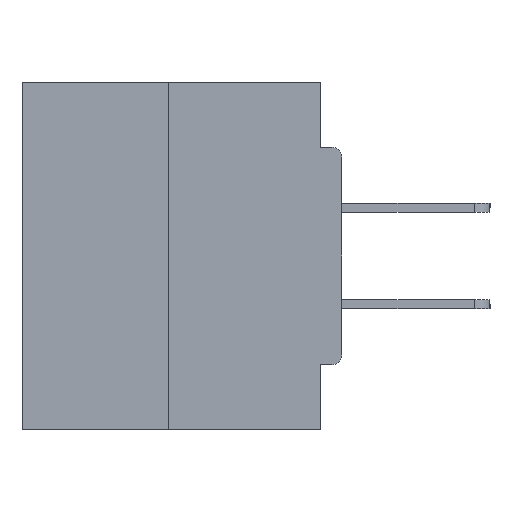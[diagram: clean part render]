
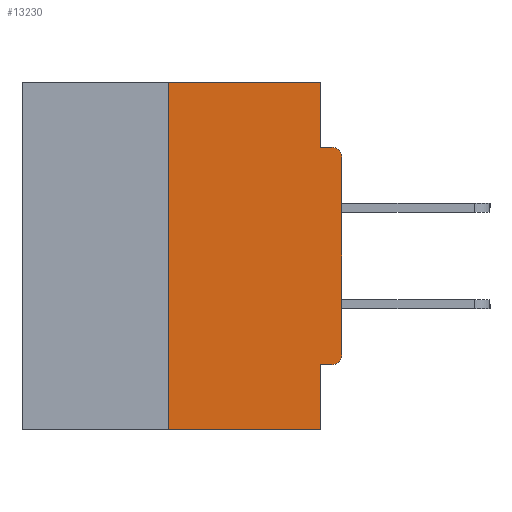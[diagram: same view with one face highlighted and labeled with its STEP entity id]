
A CAD part, left-side view. The second image highlights one B-rep face of the part: STEP entity #13230.
In plain terms, the highlighted planar face has unit normal (-1, 0, 0).
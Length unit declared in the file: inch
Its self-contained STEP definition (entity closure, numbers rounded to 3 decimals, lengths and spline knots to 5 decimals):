
#18 = VERTEX_POINT ( 'NONE', #26189 ) ;
#230 = EDGE_LOOP ( 'NONE', ( #12158, #24914, #28341, #19452, #1766, #32716, #11922, #12000, #18023, #24968 ) ) ;
#385 = VERTEX_POINT ( 'NONE', #14284 ) ;
#414 = CIRCLE ( 'NONE', #13777, 0.015 ) ;
#1766 = ORIENTED_EDGE ( 'NONE', *, *, #26395, .F. ) ;
#2534 = CARTESIAN_POINT ( 'NONE',  ( 0., 0., -0.0935 ) ) ;
#3271 = VERTEX_POINT ( 'NONE', #5292 ) ;
#3696 = CARTESIAN_POINT ( 'NONE',  ( 0., 0.46, 0. ) ) ;
#4052 = VERTEX_POINT ( 'NONE', #24921 ) ;
#4271 = VERTEX_POINT ( 'NONE', #24889 ) ;
#4394 = CARTESIAN_POINT ( 'NONE',  ( 0., 0.031, -0.4065 ) ) ;
#4814 = EDGE_CURVE ( 'NONE', #3271, #4052, #17102, .T. ) ;
#4964 = LINE ( 'NONE', #31143, #11087 ) ;
#5130 = DIRECTION ( 'NONE',  ( 0., -1., 0. ) ) ;
#5292 = CARTESIAN_POINT ( 'NONE',  ( 0., 0.015, -0.4065 ) ) ;
#5508 = CARTESIAN_POINT ( 'NONE',  ( 0., 0.031, 0. ) ) ;
#5987 = FACE_OUTER_BOUND ( 'NONE', #230, .T. ) ;
#6411 = DIRECTION ( 'NONE',  ( 0., 0., 1. ) ) ;
#7109 = DIRECTION ( 'NONE',  ( -1., 0., 0. ) ) ;
#8571 = PLANE ( 'NONE',  #15066 ) ;
#9058 = VECTOR ( 'NONE', #11011, 39.37008 ) ;
#10151 = EDGE_CURVE ( 'NONE', #31879, #18, #14123, .T. ) ;
#10481 = DIRECTION ( 'NONE',  ( 0., 0., 1. ) ) ;
#10746 = VECTOR ( 'NONE', #31750, 39.37008 ) ;
#11011 = DIRECTION ( 'NONE',  ( 0., 0., -1. ) ) ;
#11087 = VECTOR ( 'NONE', #25609, 39.37008 ) ;
#11922 = ORIENTED_EDGE ( 'NONE', *, *, #20425, .T. ) ;
#12000 = ORIENTED_EDGE ( 'NONE', *, *, #23119, .T. ) ;
#12032 = LINE ( 'NONE', #16833, #22715 ) ;
#12158 = ORIENTED_EDGE ( 'NONE', *, *, #31218, .F. ) ;
#13077 = EDGE_CURVE ( 'NONE', #14046, #31879, #32061, .T. ) ;
#13230 = ADVANCED_FACE ( 'NONE', ( #5987 ), #8571, .F. ) ;
#13777 = AXIS2_PLACEMENT_3D ( 'NONE', #22801, #7109, #25404 ) ;
#14026 = VECTOR ( 'NONE', #5130, 39.37008 ) ;
#14046 = VERTEX_POINT ( 'NONE', #24199 ) ;
#14123 = LINE ( 'NONE', #2534, #33006 ) ;
#14284 = CARTESIAN_POINT ( 'NONE',  ( 0., 0., -0.1085 ) ) ;
#14393 = DIRECTION ( 'NONE',  ( -1., 0., 0. ) ) ;
#14424 = LINE ( 'NONE', #15997, #14026 ) ;
#15066 = AXIS2_PLACEMENT_3D ( 'NONE', #3696, #26889, #29437 ) ;
#15532 = VERTEX_POINT ( 'NONE', #27314 ) ;
#15753 = DIRECTION ( 'NONE',  ( 0., -1., 0. ) ) ;
#15997 = CARTESIAN_POINT ( 'NONE',  ( 0., 0.46, 0. ) ) ;
#16410 = LINE ( 'NONE', #31680, #9058 ) ;
#16833 = CARTESIAN_POINT ( 'NONE',  ( 0., 0.46, -0.5 ) ) ;
#17102 = CIRCLE ( 'NONE', #27867, 0.015 ) ;
#18023 = ORIENTED_EDGE ( 'NONE', *, *, #10151, .F. ) ;
#18060 = VERTEX_POINT ( 'NONE', #4394 ) ;
#18352 = CARTESIAN_POINT ( 'NONE',  ( 0., 0.031, -0.0935 ) ) ;
#18541 = CARTESIAN_POINT ( 'NONE',  ( 0., 0.25, 0. ) ) ;
#19452 = ORIENTED_EDGE ( 'NONE', *, *, #33230, .F. ) ;
#20425 = EDGE_CURVE ( 'NONE', #4052, #385, #24243, .T. ) ;
#21062 = EDGE_CURVE ( 'NONE', #4271, #21348, #31194, .T. ) ;
#21348 = VERTEX_POINT ( 'NONE', #18541 ) ;
#21752 = VECTOR ( 'NONE', #6411, 39.37008 ) ;
#22088 = CARTESIAN_POINT ( 'NONE',  ( 0., 0.25, 0. ) ) ;
#22715 = VECTOR ( 'NONE', #27373, 39.37008 ) ;
#22801 = CARTESIAN_POINT ( 'NONE',  ( 0., 0.015, -0.1085 ) ) ;
#23119 = EDGE_CURVE ( 'NONE', #385, #18, #414, .T. ) ;
#24199 = CARTESIAN_POINT ( 'NONE',  ( 0., 0.031, 0. ) ) ;
#24243 = LINE ( 'NONE', #27566, #25869 ) ;
#24889 = CARTESIAN_POINT ( 'NONE',  ( 0., 0.25, -0.5 ) ) ;
#24914 = ORIENTED_EDGE ( 'NONE', *, *, #21062, .F. ) ;
#24921 = CARTESIAN_POINT ( 'NONE',  ( 0., 0., -0.3915 ) ) ;
#24968 = ORIENTED_EDGE ( 'NONE', *, *, #13077, .F. ) ;
#25404 = DIRECTION ( 'NONE',  ( 0., 0., -1. ) ) ;
#25609 = DIRECTION ( 'NONE',  ( 0., 1., 0. ) ) ;
#25869 = VECTOR ( 'NONE', #10481, 39.37008 ) ;
#26189 = CARTESIAN_POINT ( 'NONE',  ( 0., 0.015, -0.0935 ) ) ;
#26395 = EDGE_CURVE ( 'NONE', #3271, #18060, #4964, .T. ) ;
#26889 = DIRECTION ( 'NONE',  ( 1., 0., 0. ) ) ;
#27314 = CARTESIAN_POINT ( 'NONE',  ( 0., 0.031, -0.5 ) ) ;
#27373 = DIRECTION ( 'NONE',  ( 0., -1., 0. ) ) ;
#27564 = DIRECTION ( 'NONE',  ( 0., 0., -1. ) ) ;
#27566 = CARTESIAN_POINT ( 'NONE',  ( 0., 0., 0. ) ) ;
#27867 = AXIS2_PLACEMENT_3D ( 'NONE', #32954, #14393, #27564 ) ;
#28341 = ORIENTED_EDGE ( 'NONE', *, *, #30197, .T. ) ;
#29437 = DIRECTION ( 'NONE',  ( 0., 0., -1. ) ) ;
#30197 = EDGE_CURVE ( 'NONE', #4271, #15532, #12032, .T. ) ;
#31143 = CARTESIAN_POINT ( 'NONE',  ( 0., 0., -0.4065 ) ) ;
#31194 = LINE ( 'NONE', #22088, #21752 ) ;
#31218 = EDGE_CURVE ( 'NONE', #21348, #14046, #14424, .T. ) ;
#31680 = CARTESIAN_POINT ( 'NONE',  ( 0., 0.031, -0.5 ) ) ;
#31750 = DIRECTION ( 'NONE',  ( 0., 0., -1. ) ) ;
#31879 = VERTEX_POINT ( 'NONE', #18352 ) ;
#32061 = LINE ( 'NONE', #5508, #10746 ) ;
#32716 = ORIENTED_EDGE ( 'NONE', *, *, #4814, .T. ) ;
#32954 = CARTESIAN_POINT ( 'NONE',  ( 0., 0.015, -0.3915 ) ) ;
#33006 = VECTOR ( 'NONE', #15753, 39.37008 ) ;
#33230 = EDGE_CURVE ( 'NONE', #18060, #15532, #16410, .T. ) ;
